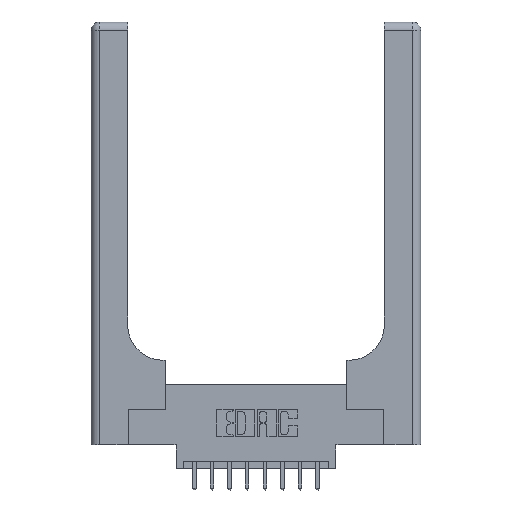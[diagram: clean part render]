
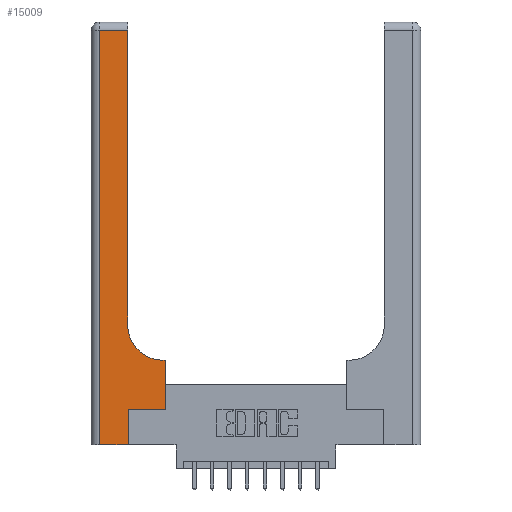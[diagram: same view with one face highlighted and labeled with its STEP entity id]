
A CAD part, top view. The second image highlights one B-rep face of the part: STEP entity #15009.
In plain terms, the highlighted planar face has unit normal (0, 0, 1).
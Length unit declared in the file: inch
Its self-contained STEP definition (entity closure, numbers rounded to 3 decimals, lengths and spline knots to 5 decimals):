
#268 = CARTESIAN_POINT ( 'NONE',  ( 0.51, 0.85, 0.37 ) ) ;
#337 = VECTOR ( 'NONE', #13216, 39.37008 ) ;
#484 = PLANE ( 'NONE',  #5830 ) ;
#643 = CARTESIAN_POINT ( 'NONE',  ( 0., 3., 0.37 ) ) ;
#712 = EDGE_CURVE ( 'NONE', #7558, #3811, #870, .T. ) ;
#870 = LINE ( 'NONE', #1406, #5317 ) ;
#1149 = CARTESIAN_POINT ( 'NONE',  ( 0., 0., 0.37 ) ) ;
#1282 = CARTESIAN_POINT ( 'NONE',  ( 0.26, 2.94, 0.37 ) ) ;
#1406 = CARTESIAN_POINT ( 'NONE',  ( 0.528, 0.25, 0.37 ) ) ;
#1411 = ORIENTED_EDGE ( 'NONE', *, *, #13138, .T. ) ;
#1528 = VERTEX_POINT ( 'NONE', #6066 ) ;
#1738 = DIRECTION ( 'NONE',  ( -1., 0., 0. ) ) ;
#1803 = ORIENTED_EDGE ( 'NONE', *, *, #712, .T. ) ;
#1867 = EDGE_CURVE ( 'NONE', #11405, #9713, #8427, .T. ) ;
#1899 = DIRECTION ( 'NONE',  ( 0., -1., 0. ) ) ;
#2160 = ORIENTED_EDGE ( 'NONE', *, *, #14398, .T. ) ;
#2213 = CARTESIAN_POINT ( 'NONE',  ( 0.265, 0.25, 0.37 ) ) ;
#2375 = ORIENTED_EDGE ( 'NONE', *, *, #1867, .T. ) ;
#2439 = ORIENTED_EDGE ( 'NONE', *, *, #9184, .T. ) ;
#2492 = EDGE_LOOP ( 'NONE', ( #2375, #2160, #7124, #1411, #2439, #10629, #1803, #6823, #12840 ) ) ;
#2688 = CARTESIAN_POINT ( 'NONE',  ( 0.51, 0.6, 0.37 ) ) ;
#3811 = VERTEX_POINT ( 'NONE', #10507 ) ;
#4547 = VECTOR ( 'NONE', #1899, 39.37008 ) ;
#4952 = CARTESIAN_POINT ( 'NONE',  ( 0.265, 0., 0.37 ) ) ;
#5044 = CARTESIAN_POINT ( 'NONE',  ( 0.265, 0.25, 0.37 ) ) ;
#5070 = DIRECTION ( 'NONE',  ( 0., 0., -1. ) ) ;
#5317 = VECTOR ( 'NONE', #9545, 39.37008 ) ;
#5730 = LINE ( 'NONE', #9375, #7911 ) ;
#5830 = AXIS2_PLACEMENT_3D ( 'NONE', #643, #12867, #12717 ) ;
#6066 = CARTESIAN_POINT ( 'NONE',  ( 0.06, 0., 0.37 ) ) ;
#6499 = CARTESIAN_POINT ( 'NONE',  ( 0.528, 0.25, 0.37 ) ) ;
#6725 = FACE_OUTER_BOUND ( 'NONE', #2492, .T. ) ;
#6823 = ORIENTED_EDGE ( 'NONE', *, *, #15401, .T. ) ;
#6971 = CARTESIAN_POINT ( 'NONE',  ( 0.26, 3., 0.37 ) ) ;
#7009 = CARTESIAN_POINT ( 'NONE',  ( 0., 2.94, 0.37 ) ) ;
#7124 = ORIENTED_EDGE ( 'NONE', *, *, #13742, .T. ) ;
#7219 = LINE ( 'NONE', #1149, #15094 ) ;
#7378 = CIRCLE ( 'NONE', #14664, 0.25 ) ;
#7558 = VERTEX_POINT ( 'NONE', #6499 ) ;
#7716 = EDGE_CURVE ( 'NONE', #7749, #7558, #8074, .T. ) ;
#7749 = VERTEX_POINT ( 'NONE', #5044 ) ;
#7911 = VECTOR ( 'NONE', #10563, 39.37008 ) ;
#7914 = VECTOR ( 'NONE', #8162, 39.37008 ) ;
#8074 = LINE ( 'NONE', #2213, #7914 ) ;
#8127 = CARTESIAN_POINT ( 'NONE',  ( 0.26, 0.85, 0.37 ) ) ;
#8162 = DIRECTION ( 'NONE',  ( 1., 0., 0. ) ) ;
#8427 = LINE ( 'NONE', #6971, #337 ) ;
#8625 = EDGE_CURVE ( 'NONE', #11265, #11405, #7378, .T. ) ;
#9184 = EDGE_CURVE ( 'NONE', #10296, #7749, #5730, .T. ) ;
#9230 = DIRECTION ( 'NONE',  ( -1., 0., 0. ) ) ;
#9375 = CARTESIAN_POINT ( 'NONE',  ( 0.265, 0., 0.37 ) ) ;
#9545 = DIRECTION ( 'NONE',  ( 0., 1., 0. ) ) ;
#9713 = VERTEX_POINT ( 'NONE', #1282 ) ;
#9907 = DIRECTION ( 'NONE',  ( 1., 0., 0. ) ) ;
#10296 = VERTEX_POINT ( 'NONE', #4952 ) ;
#10451 = LINE ( 'NONE', #12778, #4547 ) ;
#10507 = CARTESIAN_POINT ( 'NONE',  ( 0.528, 0.6, 0.37 ) ) ;
#10563 = DIRECTION ( 'NONE',  ( 0., 1., 0. ) ) ;
#10629 = ORIENTED_EDGE ( 'NONE', *, *, #7716, .T. ) ;
#10735 = LINE ( 'NONE', #7009, #14635 ) ;
#10785 = DIRECTION ( 'NONE',  ( 1., 0., 0. ) ) ;
#11265 = VERTEX_POINT ( 'NONE', #2688 ) ;
#11355 = VERTEX_POINT ( 'NONE', #13563 ) ;
#11405 = VERTEX_POINT ( 'NONE', #8127 ) ;
#12545 = CARTESIAN_POINT ( 'NONE',  ( 0.26, 0.6, 0.37 ) ) ;
#12647 = VECTOR ( 'NONE', #1738, 39.37008 ) ;
#12717 = DIRECTION ( 'NONE',  ( -1., 0., 0. ) ) ;
#12778 = CARTESIAN_POINT ( 'NONE',  ( 0.06, 3., 0.37 ) ) ;
#12840 = ORIENTED_EDGE ( 'NONE', *, *, #8625, .T. ) ;
#12867 = DIRECTION ( 'NONE',  ( 0., 0., -1. ) ) ;
#13138 = EDGE_CURVE ( 'NONE', #1528, #10296, #7219, .T. ) ;
#13216 = DIRECTION ( 'NONE',  ( 0., 1., 0. ) ) ;
#13563 = CARTESIAN_POINT ( 'NONE',  ( 0.06, 2.94, 0.37 ) ) ;
#13741 = LINE ( 'NONE', #12545, #12647 ) ;
#13742 = EDGE_CURVE ( 'NONE', #11355, #1528, #10451, .T. ) ;
#14398 = EDGE_CURVE ( 'NONE', #9713, #11355, #10735, .T. ) ;
#14635 = VECTOR ( 'NONE', #9230, 39.37008 ) ;
#14664 = AXIS2_PLACEMENT_3D ( 'NONE', #268, #5070, #9907 ) ;
#15009 = ADVANCED_FACE ( 'NONE', ( #6725 ), #484, .F. ) ;
#15094 = VECTOR ( 'NONE', #10785, 39.37008 ) ;
#15401 = EDGE_CURVE ( 'NONE', #3811, #11265, #13741, .T. ) ;
